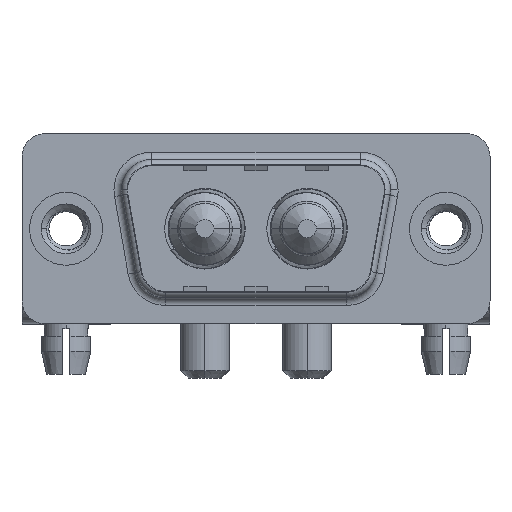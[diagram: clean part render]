
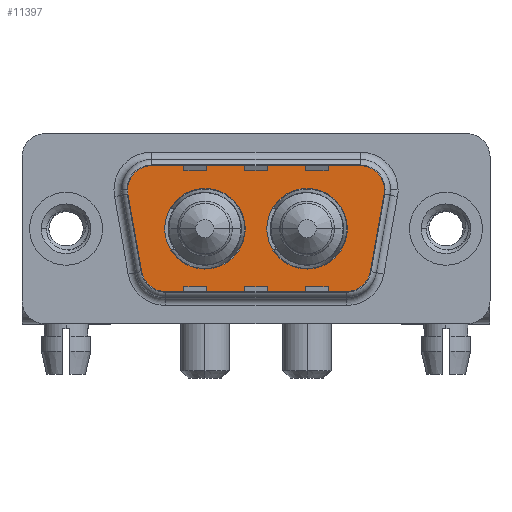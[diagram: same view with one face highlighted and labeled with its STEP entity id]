
A CAD part, top view. The second image highlights one B-rep face of the part: STEP entity #11397.
In plain terms, the highlighted planar face has unit normal (0, 0, 1).
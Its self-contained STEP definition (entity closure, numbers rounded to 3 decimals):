
#96 = CIRCLE ( 'NONE', #6856, 2. ) ;
#138 = ORIENTED_EDGE ( 'NONE', *, *, #2992, .T. ) ;
#317 = AXIS2_PLACEMENT_3D ( 'NONE', #7463, #1077, #3195 ) ;
#334 = CARTESIAN_POINT ( 'NONE',  ( 15.86, 0., 0. ) ) ;
#539 = LINE ( 'NONE', #12445, #11390 ) ;
#830 = DIRECTION ( 'NONE',  ( 0., 0., 1. ) ) ;
#1077 = DIRECTION ( 'NONE',  ( 0., 0., 1. ) ) ;
#1169 = DIRECTION ( 'NONE',  ( -1., 0., 0. ) ) ;
#1178 = CARTESIAN_POINT ( 'NONE',  ( 3.466, 2.553, 0. ) ) ;
#1228 = AXIS2_PLACEMENT_3D ( 'NONE', #6369, #11725, #10742 ) ;
#1451 = EDGE_CURVE ( 'NONE', #4816, #4566, #9981, .T. ) ;
#1452 = CIRCLE ( 'NONE', #13601, 2.65 ) ;
#1513 = DIRECTION ( 'NONE',  ( 1., 0., 0. ) ) ;
#1732 = DIRECTION ( 'NONE',  ( 1., 0., 0. ) ) ;
#1753 = CARTESIAN_POINT ( 'NONE',  ( 4.489, -3.247, 0. ) ) ;
#1810 = VERTEX_POINT ( 'NONE', #8593 ) ;
#1811 = EDGE_CURVE ( 'NONE', #1810, #6099, #96, .T. ) ;
#1896 = ORIENTED_EDGE ( 'NONE', *, *, #11238, .F. ) ;
#2019 = CARTESIAN_POINT ( 'NONE',  ( 19.564, 2.9, 0. ) ) ;
#2036 = CARTESIAN_POINT ( 'NONE',  ( 20.511, -3.247, 0. ) ) ;
#2137 = LINE ( 'NONE', #7668, #7856 ) ;
#2169 = AXIS2_PLACEMENT_3D ( 'NONE', #3869, #830, #11403 ) ;
#2346 = DIRECTION ( 'NONE',  ( 0.174, 0.985, 0. ) ) ;
#2442 = CARTESIAN_POINT ( 'NONE',  ( 18.51, 0., 0. ) ) ;
#2480 = ORIENTED_EDGE ( 'NONE', *, *, #1811, .T. ) ;
#2552 = DIRECTION ( 'NONE',  ( -1., 0., 0. ) ) ;
#2575 = DIRECTION ( 'NONE',  ( 0., 0., 1. ) ) ;
#2692 = DIRECTION ( 'NONE',  ( 0., 0., 1. ) ) ;
#2860 = CIRCLE ( 'NONE', #2169, 2.65 ) ;
#2992 = EDGE_CURVE ( 'NONE', #5587, #6135, #539, .T. ) ;
#3021 = CARTESIAN_POINT ( 'NONE',  ( 6.459, -4.9, 0. ) ) ;
#3027 = EDGE_CURVE ( 'NONE', #6512, #3628, #2860, .T. ) ;
#3030 = VERTEX_POINT ( 'NONE', #1753 ) ;
#3152 = CARTESIAN_POINT ( 'NONE',  ( 21.564, 2.9, 0. ) ) ;
#3195 = DIRECTION ( 'NONE',  ( 1., 0., 0. ) ) ;
#3302 = LINE ( 'NONE', #1178, #8522 ) ;
#3628 = VERTEX_POINT ( 'NONE', #13794 ) ;
#3731 = VERTEX_POINT ( 'NONE', #2036 ) ;
#3778 = FACE_BOUND ( 'NONE', #8708, .T. ) ;
#3854 = CARTESIAN_POINT ( 'NONE',  ( 5.436, 4.9, 0. ) ) ;
#3869 = CARTESIAN_POINT ( 'NONE',  ( 9.14, 0., 0. ) ) ;
#4114 = VECTOR ( 'NONE', #13700, 1000. ) ;
#4132 = AXIS2_PLACEMENT_3D ( 'NONE', #334, #8927, #13289 ) ;
#4151 = AXIS2_PLACEMENT_3D ( 'NONE', #11381, #2575, #1513 ) ;
#4324 = ORIENTED_EDGE ( 'NONE', *, *, #7793, .T. ) ;
#4390 = DIRECTION ( 'NONE',  ( -1., 0., 0. ) ) ;
#4406 = CARTESIAN_POINT ( 'NONE',  ( 18.541, -4.9, 0. ) ) ;
#4566 = VERTEX_POINT ( 'NONE', #6221 ) ;
#4666 = CARTESIAN_POINT ( 'NONE',  ( 6.49, 0., 0. ) ) ;
#4669 = DIRECTION ( 'NONE',  ( 0., 0., 1. ) ) ;
#4816 = VERTEX_POINT ( 'NONE', #12251 ) ;
#4826 = CIRCLE ( 'NONE', #4151, 2.65 ) ;
#4852 = DIRECTION ( 'NONE',  ( 1., 0., 0. ) ) ;
#5457 = ORIENTED_EDGE ( 'NONE', *, *, #1451, .T. ) ;
#5463 = DIRECTION ( 'NONE',  ( 0.174, -0.985, 0. ) ) ;
#5587 = VERTEX_POINT ( 'NONE', #3021 ) ;
#5778 = ORIENTED_EDGE ( 'NONE', *, *, #8019, .T. ) ;
#5796 = VERTEX_POINT ( 'NONE', #6721 ) ;
#6099 = VERTEX_POINT ( 'NONE', #3152 ) ;
#6135 = VERTEX_POINT ( 'NONE', #4406 ) ;
#6221 = CARTESIAN_POINT ( 'NONE',  ( 3.466, 2.553, 0. ) ) ;
#6369 = CARTESIAN_POINT ( 'NONE',  ( 5.436, 2.9, 0. ) ) ;
#6379 = AXIS2_PLACEMENT_3D ( 'NONE', #2019, #12990, #1169 ) ;
#6512 = VERTEX_POINT ( 'NONE', #4666 ) ;
#6721 = CARTESIAN_POINT ( 'NONE',  ( 13.21, 0., 0. ) ) ;
#6856 = AXIS2_PLACEMENT_3D ( 'NONE', #7401, #9800, #4390 ) ;
#6934 = EDGE_CURVE ( 'NONE', #4566, #3030, #3302, .T. ) ;
#7066 = FACE_OUTER_BOUND ( 'NONE', #7514, .T. ) ;
#7174 = DIRECTION ( 'NONE',  ( 1., 0., 0. ) ) ;
#7196 = ORIENTED_EDGE ( 'NONE', *, *, #13548, .T. ) ;
#7401 = CARTESIAN_POINT ( 'NONE',  ( 19.564, 2.9, 0. ) ) ;
#7463 = CARTESIAN_POINT ( 'NONE',  ( 18.541, -2.9, 0. ) ) ;
#7514 = EDGE_LOOP ( 'NONE', ( #12341, #4324, #2480, #7196, #10667, #5457, #13405, #5778, #138 ) ) ;
#7668 = CARTESIAN_POINT ( 'NONE',  ( 21.534, 2.553, 0. ) ) ;
#7697 = VERTEX_POINT ( 'NONE', #10298 ) ;
#7793 = EDGE_CURVE ( 'NONE', #3731, #1810, #2137, .T. ) ;
#7856 = VECTOR ( 'NONE', #2346, 1000. ) ;
#8019 = EDGE_CURVE ( 'NONE', #3030, #5587, #9455, .T. ) ;
#8191 = LINE ( 'NONE', #3854, #4114 ) ;
#8259 = PLANE ( 'NONE',  #317 ) ;
#8328 = AXIS2_PLACEMENT_3D ( 'NONE', #13387, #4669, #2552 ) ;
#8522 = VECTOR ( 'NONE', #5463, 1000. ) ;
#8593 = CARTESIAN_POINT ( 'NONE',  ( 21.534, 2.553, 0. ) ) ;
#8708 = EDGE_LOOP ( 'NONE', ( #12326, #10463 ) ) ;
#8927 = DIRECTION ( 'NONE',  ( 0., 0., 1. ) ) ;
#9209 = CIRCLE ( 'NONE', #10337, 2. ) ;
#9455 = CIRCLE ( 'NONE', #8328, 2. ) ;
#9488 = EDGE_CURVE ( 'NONE', #7697, #4816, #8191, .T. ) ;
#9800 = DIRECTION ( 'NONE',  ( 0., 0., 1. ) ) ;
#9981 = CIRCLE ( 'NONE', #1228, 2. ) ;
#10298 = CARTESIAN_POINT ( 'NONE',  ( 19.564, 4.9, 0. ) ) ;
#10306 = EDGE_CURVE ( 'NONE', #12206, #5796, #1452, .T. ) ;
#10337 = AXIS2_PLACEMENT_3D ( 'NONE', #10371, #11164, #1732 ) ;
#10371 = CARTESIAN_POINT ( 'NONE',  ( 18.541, -2.9, 0. ) ) ;
#10463 = ORIENTED_EDGE ( 'NONE', *, *, #10914, .F. ) ;
#10667 = ORIENTED_EDGE ( 'NONE', *, *, #9488, .T. ) ;
#10742 = DIRECTION ( 'NONE',  ( 1., 0., 0. ) ) ;
#10914 = EDGE_CURVE ( 'NONE', #5796, #12206, #13331, .T. ) ;
#11164 = DIRECTION ( 'NONE',  ( 0., 0., 1. ) ) ;
#11238 = EDGE_CURVE ( 'NONE', #3628, #6512, #4826, .T. ) ;
#11381 = CARTESIAN_POINT ( 'NONE',  ( 9.14, 0., 0. ) ) ;
#11390 = VECTOR ( 'NONE', #4852, 1000. ) ;
#11397 = ADVANCED_FACE ( 'NONE', ( #3778, #12349, #7066 ), #8259, .T. ) ;
#11403 = DIRECTION ( 'NONE',  ( 1., 0., 0. ) ) ;
#11408 = ORIENTED_EDGE ( 'NONE', *, *, #3027, .F. ) ;
#11725 = DIRECTION ( 'NONE',  ( 0., 0., 1. ) ) ;
#12181 = CARTESIAN_POINT ( 'NONE',  ( 15.86, 0., 0. ) ) ;
#12206 = VERTEX_POINT ( 'NONE', #2442 ) ;
#12251 = CARTESIAN_POINT ( 'NONE',  ( 5.436, 4.9, 0. ) ) ;
#12326 = ORIENTED_EDGE ( 'NONE', *, *, #10306, .F. ) ;
#12341 = ORIENTED_EDGE ( 'NONE', *, *, #12385, .T. ) ;
#12349 = FACE_BOUND ( 'NONE', #13287, .T. ) ;
#12385 = EDGE_CURVE ( 'NONE', #6135, #3731, #9209, .T. ) ;
#12445 = CARTESIAN_POINT ( 'NONE',  ( 6.459, -4.9, 0. ) ) ;
#12990 = DIRECTION ( 'NONE',  ( 0., 0., 1. ) ) ;
#13287 = EDGE_LOOP ( 'NONE', ( #1896, #11408 ) ) ;
#13289 = DIRECTION ( 'NONE',  ( 1., 0., 0. ) ) ;
#13331 = CIRCLE ( 'NONE', #4132, 2.65 ) ;
#13387 = CARTESIAN_POINT ( 'NONE',  ( 6.459, -2.9, 0. ) ) ;
#13405 = ORIENTED_EDGE ( 'NONE', *, *, #6934, .T. ) ;
#13548 = EDGE_CURVE ( 'NONE', #6099, #7697, #13804, .T. ) ;
#13601 = AXIS2_PLACEMENT_3D ( 'NONE', #12181, #2692, #7174 ) ;
#13700 = DIRECTION ( 'NONE',  ( -1., 0., 0. ) ) ;
#13794 = CARTESIAN_POINT ( 'NONE',  ( 11.79, 0., 0. ) ) ;
#13804 = CIRCLE ( 'NONE', #6379, 2. ) ;
